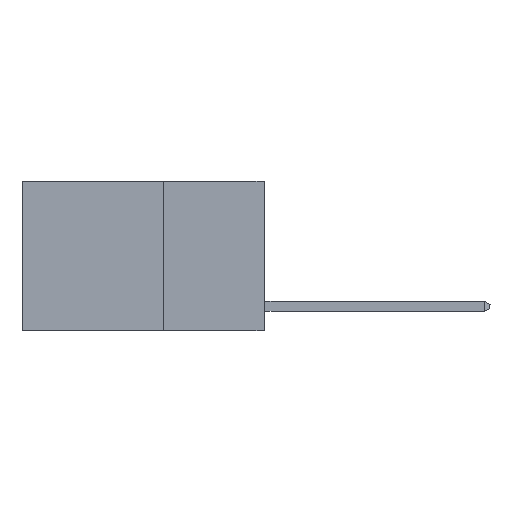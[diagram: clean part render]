
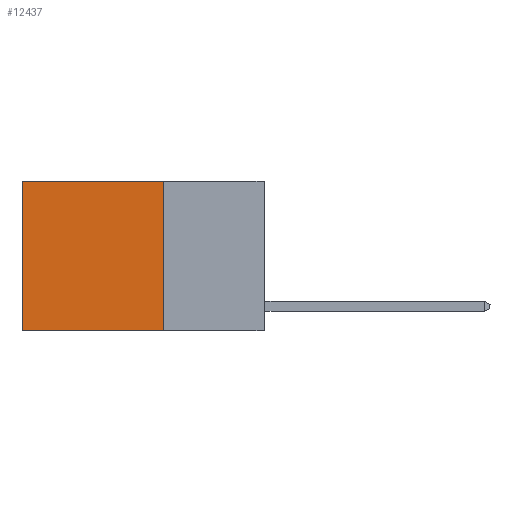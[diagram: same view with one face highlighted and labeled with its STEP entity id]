
A CAD part, left-side view. The second image highlights one B-rep face of the part: STEP entity #12437.
In plain terms, the highlighted planar face has unit normal (-1, 0, 0).
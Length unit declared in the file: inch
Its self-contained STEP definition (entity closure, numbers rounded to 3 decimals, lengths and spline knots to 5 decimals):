
#504 = VECTOR ( 'NONE', #5922, 39.37008 ) ;
#1048 = VECTOR ( 'NONE', #22285, 39.37008 ) ;
#1369 = ORIENTED_EDGE ( 'NONE', *, *, #25262, .T. ) ;
#1948 = DIRECTION ( 'NONE',  ( 1., 0., 0. ) ) ;
#3568 = CARTESIAN_POINT ( 'NONE',  ( 0.2625, 0.6, 0. ) ) ;
#5909 = VERTEX_POINT ( 'NONE', #6037 ) ;
#5922 = DIRECTION ( 'NONE',  ( 0., 1., 0. ) ) ;
#6037 = CARTESIAN_POINT ( 'NONE',  ( 0.2625, 0.25, -0.37 ) ) ;
#7495 = DIRECTION ( 'NONE',  ( 0., 1., 0. ) ) ;
#8020 = LINE ( 'NONE', #26612, #22399 ) ;
#8219 = CARTESIAN_POINT ( 'NONE',  ( 0.2625, 0.25, 0. ) ) ;
#8492 = FACE_OUTER_BOUND ( 'NONE', #21984, .T. ) ;
#9815 = CARTESIAN_POINT ( 'NONE',  ( 0.2625, 0.6, 0. ) ) ;
#10187 = CARTESIAN_POINT ( 'NONE',  ( 0.2625, 0.6, -0.37 ) ) ;
#10777 = LINE ( 'NONE', #19211, #11677 ) ;
#11357 = AXIS2_PLACEMENT_3D ( 'NONE', #8219, #1948, #14545 ) ;
#11677 = VECTOR ( 'NONE', #17021, 39.37008 ) ;
#12382 = LINE ( 'NONE', #24777, #504 ) ;
#12437 = ADVANCED_FACE ( 'NONE', ( #8492 ), #25024, .F. ) ;
#13964 = LINE ( 'NONE', #3568, #1048 ) ;
#14345 = VERTEX_POINT ( 'NONE', #10187 ) ;
#14545 = DIRECTION ( 'NONE',  ( 0., 0., -1. ) ) ;
#15739 = VERTEX_POINT ( 'NONE', #9815 ) ;
#16360 = EDGE_CURVE ( 'NONE', #5909, #14345, #12382, .T. ) ;
#16384 = ORIENTED_EDGE ( 'NONE', *, *, #16360, .F. ) ;
#17021 = DIRECTION ( 'NONE',  ( 0., 0., -1. ) ) ;
#18031 = VERTEX_POINT ( 'NONE', #19999 ) ;
#18558 = EDGE_CURVE ( 'NONE', #15739, #14345, #13964, .T. ) ;
#19211 = CARTESIAN_POINT ( 'NONE',  ( 0.2625, 0.25, 0. ) ) ;
#19999 = CARTESIAN_POINT ( 'NONE',  ( 0.2625, 0.25, 0. ) ) ;
#21984 = EDGE_LOOP ( 'NONE', ( #23397, #16384, #22017, #1369 ) ) ;
#22017 = ORIENTED_EDGE ( 'NONE', *, *, #22061, .F. ) ;
#22061 = EDGE_CURVE ( 'NONE', #18031, #5909, #10777, .T. ) ;
#22285 = DIRECTION ( 'NONE',  ( 0., 0., -1. ) ) ;
#22399 = VECTOR ( 'NONE', #7495, 39.37008 ) ;
#23397 = ORIENTED_EDGE ( 'NONE', *, *, #18558, .T. ) ;
#24777 = CARTESIAN_POINT ( 'NONE',  ( 0.2625, 0.25, -0.37 ) ) ;
#25024 = PLANE ( 'NONE',  #11357 ) ;
#25262 = EDGE_CURVE ( 'NONE', #18031, #15739, #8020, .T. ) ;
#26612 = CARTESIAN_POINT ( 'NONE',  ( 0.2625, 0.25, 0. ) ) ;
